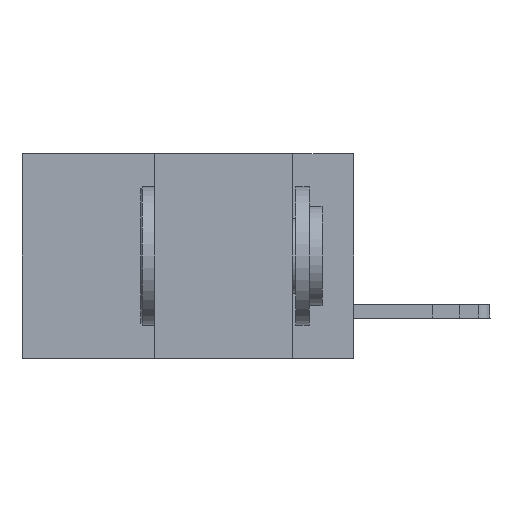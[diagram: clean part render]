
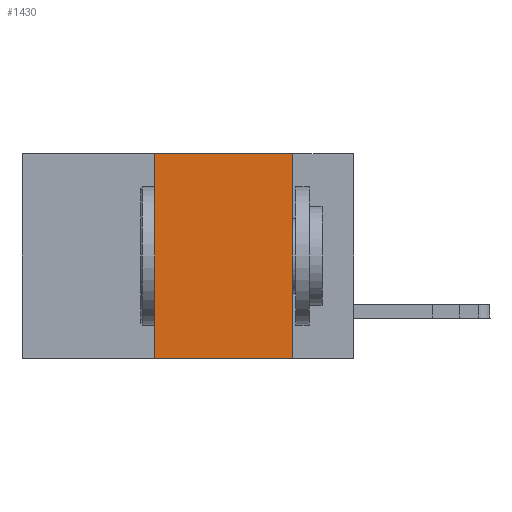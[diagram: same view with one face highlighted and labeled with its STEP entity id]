
A CAD part, left-side view. The second image highlights one B-rep face of the part: STEP entity #1430.
In plain terms, the highlighted planar face has unit normal (-1, 0, 0).
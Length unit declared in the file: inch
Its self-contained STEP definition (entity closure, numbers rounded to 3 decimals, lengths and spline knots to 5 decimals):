
#536 = DIRECTION ( 'NONE',  ( 0., 0., 1. ) ) ;
#779 = DIRECTION ( 'NONE',  ( 0., 0., -1. ) ) ;
#907 = VERTEX_POINT ( 'NONE', #5390 ) ;
#1283 = ORIENTED_EDGE ( 'NONE', *, *, #1693, .F. ) ;
#1411 = VECTOR ( 'NONE', #14372, 39.37008 ) ;
#1430 = ADVANCED_FACE ( 'NONE', ( #14050 ), #6559, .F. ) ;
#1575 = CARTESIAN_POINT ( 'NONE',  ( 0., 0.11, 0. ) ) ;
#1693 = EDGE_CURVE ( 'NONE', #12686, #907, #2350, .T. ) ;
#2350 = LINE ( 'NONE', #2680, #1411 ) ;
#2680 = CARTESIAN_POINT ( 'NONE',  ( 0., 0.11, 0. ) ) ;
#2792 = AXIS2_PLACEMENT_3D ( 'NONE', #7872, #18085, #779 ) ;
#3874 = EDGE_CURVE ( 'NONE', #6351, #12686, #18661, .T. ) ;
#5390 = CARTESIAN_POINT ( 'NONE',  ( 0., 0.11, -0.37 ) ) ;
#5792 = VECTOR ( 'NONE', #7044, 39.37008 ) ;
#6173 = CARTESIAN_POINT ( 'NONE',  ( 0., 0.36, -0.37 ) ) ;
#6351 = VERTEX_POINT ( 'NONE', #12179 ) ;
#6559 = PLANE ( 'NONE',  #2792 ) ;
#7044 = DIRECTION ( 'NONE',  ( 0., -1., 0. ) ) ;
#7099 = ORIENTED_EDGE ( 'NONE', *, *, #3874, .F. ) ;
#7872 = CARTESIAN_POINT ( 'NONE',  ( 0., 0.6, 0. ) ) ;
#8948 = EDGE_CURVE ( 'NONE', #18018, #6351, #18738, .T. ) ;
#10641 = DIRECTION ( 'NONE',  ( 0., -1., 0. ) ) ;
#11689 = ORIENTED_EDGE ( 'NONE', *, *, #17994, .T. ) ;
#12179 = CARTESIAN_POINT ( 'NONE',  ( 0., 0.36, 0. ) ) ;
#12686 = VERTEX_POINT ( 'NONE', #1575 ) ;
#13609 = VECTOR ( 'NONE', #10641, 39.37008 ) ;
#14050 = FACE_OUTER_BOUND ( 'NONE', #14892, .T. ) ;
#14202 = CARTESIAN_POINT ( 'NONE',  ( 0., 0.6, 0. ) ) ;
#14372 = DIRECTION ( 'NONE',  ( 0., 0., -1. ) ) ;
#14892 = EDGE_LOOP ( 'NONE', ( #1283, #7099, #17116, #11689 ) ) ;
#15410 = LINE ( 'NONE', #16326, #13609 ) ;
#15977 = VECTOR ( 'NONE', #536, 39.37008 ) ;
#16326 = CARTESIAN_POINT ( 'NONE',  ( 0., 0.6, -0.37 ) ) ;
#16491 = CARTESIAN_POINT ( 'NONE',  ( 0., 0.36, 0. ) ) ;
#17116 = ORIENTED_EDGE ( 'NONE', *, *, #8948, .F. ) ;
#17994 = EDGE_CURVE ( 'NONE', #18018, #907, #15410, .T. ) ;
#18018 = VERTEX_POINT ( 'NONE', #6173 ) ;
#18085 = DIRECTION ( 'NONE',  ( 1., 0., 0. ) ) ;
#18661 = LINE ( 'NONE', #14202, #5792 ) ;
#18738 = LINE ( 'NONE', #16491, #15977 ) ;
